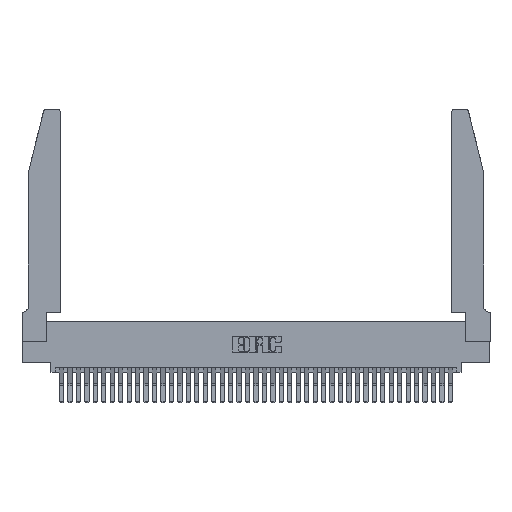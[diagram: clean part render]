
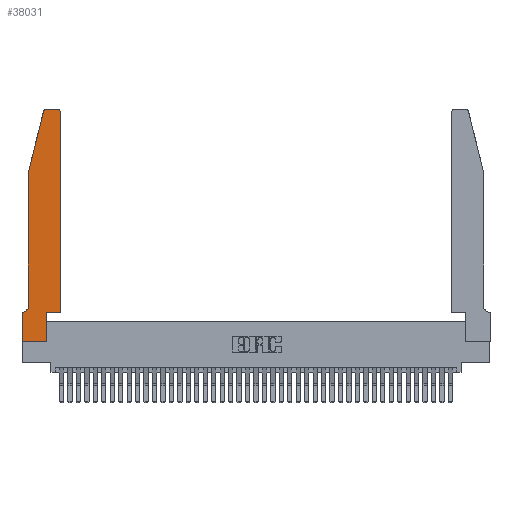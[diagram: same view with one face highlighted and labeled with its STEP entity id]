
A CAD part, top view. The second image highlights one B-rep face of the part: STEP entity #38031.
In plain terms, the highlighted planar face has unit normal (0, 0, 1).
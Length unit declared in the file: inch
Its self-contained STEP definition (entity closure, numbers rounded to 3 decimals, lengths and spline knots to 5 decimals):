
#101 = ORIENTED_EDGE ( 'NONE', *, *, #34549, .T. ) ;
#513 = DIRECTION ( 'NONE',  ( 0., 1., 0. ) ) ;
#687 = ORIENTED_EDGE ( 'NONE', *, *, #11803, .T. ) ;
#693 = DIRECTION ( 'NONE',  ( 0., -1., 0. ) ) ;
#714 = CARTESIAN_POINT ( 'NONE',  ( 0.2865, 0.35, 0.37 ) ) ;
#751 = EDGE_CURVE ( 'NONE', #17487, #4416, #24046, .T. ) ;
#1165 = DIRECTION ( 'NONE',  ( 1., 0., 0. ) ) ;
#1616 = EDGE_CURVE ( 'NONE', #14676, #28557, #25937, .T. ) ;
#1982 = CARTESIAN_POINT ( 'NONE',  ( 0., 0.35, 0.37 ) ) ;
#2309 = EDGE_CURVE ( 'NONE', #28557, #18508, #27341, .T. ) ;
#2467 = ORIENTED_EDGE ( 'NONE', *, *, #29166, .T. ) ;
#2774 = ORIENTED_EDGE ( 'NONE', *, *, #34725, .T. ) ;
#3969 = EDGE_CURVE ( 'NONE', #18508, #25676, #40137, .T. ) ;
#4232 = ORIENTED_EDGE ( 'NONE', *, *, #36064, .T. ) ;
#4416 = VERTEX_POINT ( 'NONE', #12649 ) ;
#4460 = EDGE_CURVE ( 'NONE', #21595, #9971, #33692, .T. ) ;
#4515 = CARTESIAN_POINT ( 'NONE',  ( 0.0055, 0.42, 0.37 ) ) ;
#4564 = VERTEX_POINT ( 'NONE', #37707 ) ;
#4751 = AXIS2_PLACEMENT_3D ( 'NONE', #18201, #39765, #21003 ) ;
#5738 = ORIENTED_EDGE ( 'NONE', *, *, #2309, .T. ) ;
#5794 = CARTESIAN_POINT ( 'NONE',  ( 0., 0., 0.37 ) ) ;
#6742 = DIRECTION ( 'NONE',  ( -1., 0., 0. ) ) ;
#7024 = DIRECTION ( 'NONE',  ( 1., 0., 0. ) ) ;
#7311 = EDGE_LOOP ( 'NONE', ( #10684, #4232, #2467, #16920, #23382, #101, #2774, #14604, #5738, #27634, #687, #22996 ) ) ;
#7315 = DIRECTION ( 'NONE',  ( -1., 0., 0. ) ) ;
#7651 = PLANE ( 'NONE',  #18293 ) ;
#8278 = VECTOR ( 'NONE', #7024, 39.37008 ) ;
#8581 = FACE_OUTER_BOUND ( 'NONE', #7311, .T. ) ;
#8972 = VECTOR ( 'NONE', #12200, 39.37008 ) ;
#9079 = CARTESIAN_POINT ( 'NONE',  ( 0.4505, 0.35, 0.37 ) ) ;
#9803 = VECTOR ( 'NONE', #6742, 39.37008 ) ;
#9971 = VERTEX_POINT ( 'NONE', #39569 ) ;
#10449 = CARTESIAN_POINT ( 'NONE',  ( 0., 0.35, 0.37 ) ) ;
#10665 = DIRECTION ( 'NONE',  ( 0., 0., 1. ) ) ;
#10684 = ORIENTED_EDGE ( 'NONE', *, *, #21681, .T. ) ;
#10879 = CARTESIAN_POINT ( 'NONE',  ( 0.0755, 2., 0.37 ) ) ;
#11803 = EDGE_CURVE ( 'NONE', #25676, #21595, #29005, .T. ) ;
#12200 = DIRECTION ( 'NONE',  ( -1., 0., 0. ) ) ;
#12401 = VECTOR ( 'NONE', #513, 39.37008 ) ;
#12649 = CARTESIAN_POINT ( 'NONE',  ( 0.0755, 0.42, 0.37 ) ) ;
#12961 = LINE ( 'NONE', #31260, #8972 ) ;
#13387 = CARTESIAN_POINT ( 'NONE',  ( 0., 0., 0.37 ) ) ;
#14414 = DIRECTION ( 'NONE',  ( 1., 0., 0. ) ) ;
#14526 = AXIS2_PLACEMENT_3D ( 'NONE', #23064, #10665, #1165 ) ;
#14604 = ORIENTED_EDGE ( 'NONE', *, *, #1616, .T. ) ;
#14676 = VERTEX_POINT ( 'NONE', #5794 ) ;
#15927 = CARTESIAN_POINT ( 'NONE',  ( 0.0755, 0.35, 0.37 ) ) ;
#16920 = ORIENTED_EDGE ( 'NONE', *, *, #751, .T. ) ;
#17487 = VERTEX_POINT ( 'NONE', #22394 ) ;
#18201 = CARTESIAN_POINT ( 'NONE',  ( 0.4205, 2.72, 0.37 ) ) ;
#18293 = AXIS2_PLACEMENT_3D ( 'NONE', #10449, #39088, #32998 ) ;
#18508 = VERTEX_POINT ( 'NONE', #714 ) ;
#19349 = CIRCLE ( 'NONE', #24580, 0.07 ) ;
#21003 = DIRECTION ( 'NONE',  ( 1., 0., 0. ) ) ;
#21328 = VECTOR ( 'NONE', #693, 39.37008 ) ;
#21595 = VERTEX_POINT ( 'NONE', #24617 ) ;
#21681 = EDGE_CURVE ( 'NONE', #9971, #4564, #12961, .T. ) ;
#22394 = CARTESIAN_POINT ( 'NONE',  ( 0.0755, 2., 0.37 ) ) ;
#22996 = ORIENTED_EDGE ( 'NONE', *, *, #4460, .T. ) ;
#23044 = VECTOR ( 'NONE', #33143, 39.37008 ) ;
#23064 = CARTESIAN_POINT ( 'NONE',  ( 0.284, 2.72, 0.37 ) ) ;
#23382 = ORIENTED_EDGE ( 'NONE', *, *, #33336, .T. ) ;
#23619 = CARTESIAN_POINT ( 'NONE',  ( 0., 0., 0.37 ) ) ;
#24046 = LINE ( 'NONE', #32148, #36943 ) ;
#24580 = AXIS2_PLACEMENT_3D ( 'NONE', #4515, #39605, #7315 ) ;
#24617 = CARTESIAN_POINT ( 'NONE',  ( 0.4505, 2.72, 0.37 ) ) ;
#25556 = LINE ( 'NONE', #10879, #23044 ) ;
#25676 = VERTEX_POINT ( 'NONE', #9079 ) ;
#25937 = LINE ( 'NONE', #23619, #39858 ) ;
#26533 = VECTOR ( 'NONE', #32669, 39.37008 ) ;
#26793 = LINE ( 'NONE', #13387, #21328 ) ;
#27341 = LINE ( 'NONE', #32392, #12401 ) ;
#27634 = ORIENTED_EDGE ( 'NONE', *, *, #3969, .T. ) ;
#28040 = CARTESIAN_POINT ( 'NONE',  ( 0.0055, 0.35, 0.37 ) ) ;
#28557 = VERTEX_POINT ( 'NONE', #39099 ) ;
#28811 = VERTEX_POINT ( 'NONE', #1982 ) ;
#29005 = LINE ( 'NONE', #29594, #26533 ) ;
#29166 = EDGE_CURVE ( 'NONE', #40418, #17487, #25556, .T. ) ;
#29594 = CARTESIAN_POINT ( 'NONE',  ( 0.4505, 0.35, 0.37 ) ) ;
#31260 = CARTESIAN_POINT ( 'NONE',  ( 0.2605, 2.75, 0.37 ) ) ;
#31712 = LINE ( 'NONE', #15927, #9803 ) ;
#32148 = CARTESIAN_POINT ( 'NONE',  ( 0.0755, 2., 0.37 ) ) ;
#32392 = CARTESIAN_POINT ( 'NONE',  ( 0.2865, 0.35, 0.37 ) ) ;
#32669 = DIRECTION ( 'NONE',  ( 0., 1., 0. ) ) ;
#32998 = DIRECTION ( 'NONE',  ( 1., 0., 0. ) ) ;
#33143 = DIRECTION ( 'NONE',  ( -0.239, -0.971, 0. ) ) ;
#33336 = EDGE_CURVE ( 'NONE', #4416, #33619, #19349, .T. ) ;
#33619 = VERTEX_POINT ( 'NONE', #28040 ) ;
#33692 = CIRCLE ( 'NONE', #4751, 0.03 ) ;
#34549 = EDGE_CURVE ( 'NONE', #33619, #28811, #31712, .T. ) ;
#34725 = EDGE_CURVE ( 'NONE', #28811, #14676, #26793, .T. ) ;
#36064 = EDGE_CURVE ( 'NONE', #4564, #40418, #38584, .T. ) ;
#36943 = VECTOR ( 'NONE', #39080, 39.37008 ) ;
#37707 = CARTESIAN_POINT ( 'NONE',  ( 0.284, 2.75, 0.37 ) ) ;
#38031 = ADVANCED_FACE ( 'NONE', ( #8581 ), #7651, .T. ) ;
#38072 = CARTESIAN_POINT ( 'NONE',  ( 0.4505, 0.35, 0.37 ) ) ;
#38584 = CIRCLE ( 'NONE', #14526, 0.03 ) ;
#39080 = DIRECTION ( 'NONE',  ( 0., -1., 0. ) ) ;
#39088 = DIRECTION ( 'NONE',  ( 0., 0., 1. ) ) ;
#39099 = CARTESIAN_POINT ( 'NONE',  ( 0.2865, 0., 0.37 ) ) ;
#39333 = CARTESIAN_POINT ( 'NONE',  ( 0.25487, 2.72718, 0.37 ) ) ;
#39569 = CARTESIAN_POINT ( 'NONE',  ( 0.4205, 2.75, 0.37 ) ) ;
#39605 = DIRECTION ( 'NONE',  ( 0., 0., -1. ) ) ;
#39765 = DIRECTION ( 'NONE',  ( 0., 0., 1. ) ) ;
#39858 = VECTOR ( 'NONE', #14414, 39.37008 ) ;
#40137 = LINE ( 'NONE', #38072, #8278 ) ;
#40418 = VERTEX_POINT ( 'NONE', #39333 ) ;
